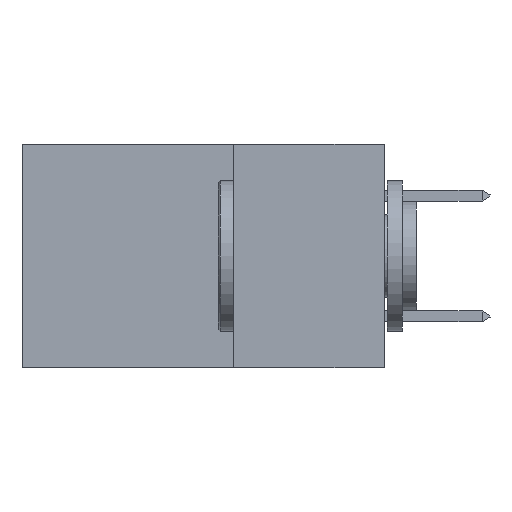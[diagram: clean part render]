
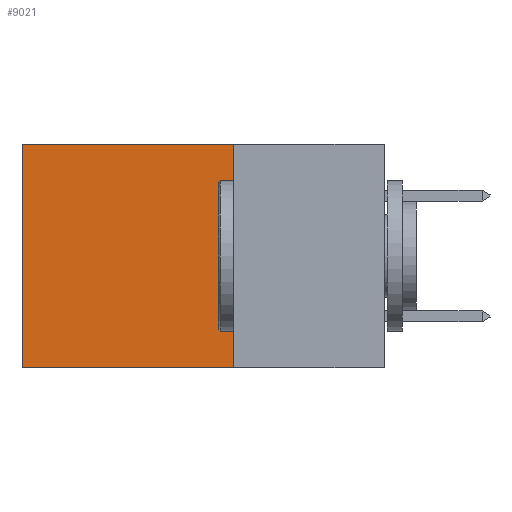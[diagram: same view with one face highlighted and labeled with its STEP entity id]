
A CAD part, left-side view. The second image highlights one B-rep face of the part: STEP entity #9021.
In plain terms, the highlighted planar face has unit normal (-1, 0, 0).
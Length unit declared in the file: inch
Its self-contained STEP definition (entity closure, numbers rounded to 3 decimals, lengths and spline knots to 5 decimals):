
#242 = CARTESIAN_POINT ( 'NONE',  ( 0.2875, 0.6, 0. ) ) ;
#490 = VERTEX_POINT ( 'NONE', #12384 ) ;
#1016 = AXIS2_PLACEMENT_3D ( 'NONE', #24931, #10581, #12992 ) ;
#2993 = FACE_OUTER_BOUND ( 'NONE', #9067, .T. ) ;
#4992 = DIRECTION ( 'NONE',  ( 0., 0., -1. ) ) ;
#6125 = ORIENTED_EDGE ( 'NONE', *, *, #25685, .T. ) ;
#7105 = EDGE_CURVE ( 'NONE', #22002, #18244, #20210, .T. ) ;
#7427 = VECTOR ( 'NONE', #4992, 39.37008 ) ;
#8363 = ORIENTED_EDGE ( 'NONE', *, *, #22333, .F. ) ;
#8399 = ORIENTED_EDGE ( 'NONE', *, *, #7105, .T. ) ;
#9021 = ADVANCED_FACE ( 'NONE', ( #2993 ), #18048, .F. ) ;
#9067 = EDGE_LOOP ( 'NONE', ( #8399, #26877, #8363, #6125 ) ) ;
#10581 = DIRECTION ( 'NONE',  ( 1., 0., 0. ) ) ;
#11394 = CARTESIAN_POINT ( 'NONE',  ( 0.2875, 0.25, -0.37 ) ) ;
#12334 = VERTEX_POINT ( 'NONE', #11394 ) ;
#12384 = CARTESIAN_POINT ( 'NONE',  ( 0.2875, 0.25, 0. ) ) ;
#12992 = DIRECTION ( 'NONE',  ( 0., 0., -1. ) ) ;
#14036 = LINE ( 'NONE', #14638, #29390 ) ;
#14638 = CARTESIAN_POINT ( 'NONE',  ( 0.2875, 0.25, 0. ) ) ;
#15458 = LINE ( 'NONE', #16364, #28941 ) ;
#16057 = VECTOR ( 'NONE', #31067, 39.37008 ) ;
#16364 = CARTESIAN_POINT ( 'NONE',  ( 0.2875, 0.25, 0. ) ) ;
#16791 = CARTESIAN_POINT ( 'NONE',  ( 0.2875, 0.25, -0.37 ) ) ;
#18048 = PLANE ( 'NONE',  #1016 ) ;
#18244 = VERTEX_POINT ( 'NONE', #22591 ) ;
#20210 = LINE ( 'NONE', #242, #7427 ) ;
#22002 = VERTEX_POINT ( 'NONE', #25104 ) ;
#22333 = EDGE_CURVE ( 'NONE', #490, #12334, #14036, .T. ) ;
#22591 = CARTESIAN_POINT ( 'NONE',  ( 0.2875, 0.6, -0.37 ) ) ;
#24231 = LINE ( 'NONE', #16791, #16057 ) ;
#24931 = CARTESIAN_POINT ( 'NONE',  ( 0.2875, 0.25, 0. ) ) ;
#25104 = CARTESIAN_POINT ( 'NONE',  ( 0.2875, 0.6, 0. ) ) ;
#25685 = EDGE_CURVE ( 'NONE', #490, #22002, #15458, .T. ) ;
#26877 = ORIENTED_EDGE ( 'NONE', *, *, #28250, .F. ) ;
#28250 = EDGE_CURVE ( 'NONE', #12334, #18244, #24231, .T. ) ;
#28276 = DIRECTION ( 'NONE',  ( 0., 1., 0. ) ) ;
#28941 = VECTOR ( 'NONE', #28276, 39.37008 ) ;
#29078 = DIRECTION ( 'NONE',  ( 0., 0., -1. ) ) ;
#29390 = VECTOR ( 'NONE', #29078, 39.37008 ) ;
#31067 = DIRECTION ( 'NONE',  ( 0., 1., 0. ) ) ;
